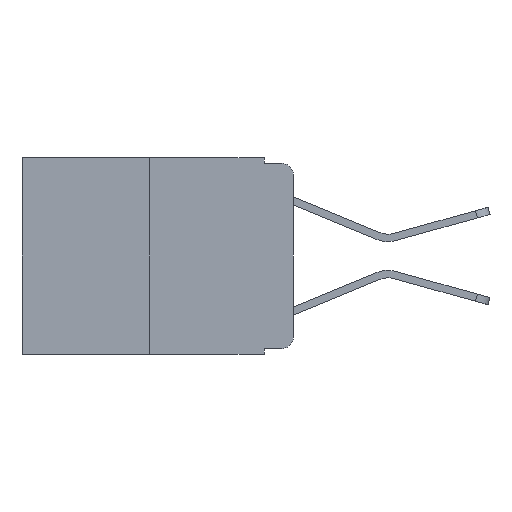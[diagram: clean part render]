
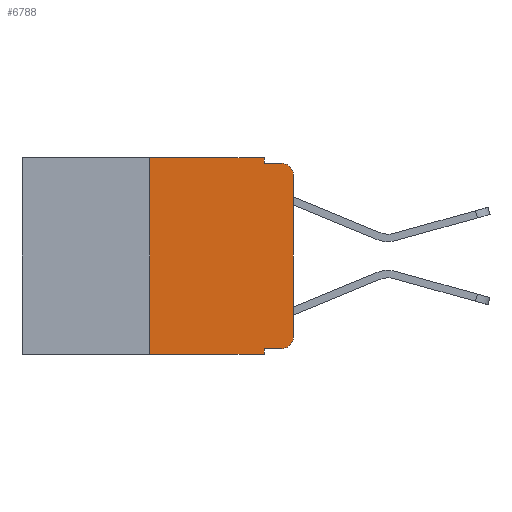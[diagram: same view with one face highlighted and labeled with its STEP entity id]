
A CAD part, left-side view. The second image highlights one B-rep face of the part: STEP entity #6788.
In plain terms, the highlighted planar face has unit normal (-1, 0, 0).
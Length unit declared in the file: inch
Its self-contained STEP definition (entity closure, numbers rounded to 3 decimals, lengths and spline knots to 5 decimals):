
#17 = DIRECTION ( 'NONE',  ( 1., 0., 0. ) ) ;
#64 = ORIENTED_EDGE ( 'NONE', *, *, #7757, .T. ) ;
#306 = CARTESIAN_POINT ( 'NONE',  ( 0., 0.02, -0.313 ) ) ;
#849 = ORIENTED_EDGE ( 'NONE', *, *, #4916, .T. ) ;
#918 = LINE ( 'NONE', #1607, #7375 ) ;
#1064 = AXIS2_PLACEMENT_3D ( 'NONE', #2397, #3170, #8493 ) ;
#1242 = DIRECTION ( 'NONE',  ( 0., -1., 0. ) ) ;
#1512 = EDGE_CURVE ( 'NONE', #9832, #6600, #7458, .T. ) ;
#1607 = CARTESIAN_POINT ( 'NONE',  ( 0., 0.473, 0. ) ) ;
#1700 = LINE ( 'NONE', #7410, #6364 ) ;
#1764 = DIRECTION ( 'NONE',  ( -1., 0., 0. ) ) ;
#1778 = ORIENTED_EDGE ( 'NONE', *, *, #9195, .F. ) ;
#2038 = LINE ( 'NONE', #7457, #3850 ) ;
#2186 = EDGE_CURVE ( 'NONE', #6170, #4249, #1700, .T. ) ;
#2193 = CARTESIAN_POINT ( 'NONE',  ( 0., 0.25, -0.343 ) ) ;
#2313 = VECTOR ( 'NONE', #8020, 39.37008 ) ;
#2341 = EDGE_CURVE ( 'NONE', #6851, #3588, #7324, .T. ) ;
#2349 = VERTEX_POINT ( 'NONE', #8734 ) ;
#2397 = CARTESIAN_POINT ( 'NONE',  ( 0., 0.02, -0.03 ) ) ;
#2400 = CARTESIAN_POINT ( 'NONE',  ( 0., 0.051, 0. ) ) ;
#2584 = CARTESIAN_POINT ( 'NONE',  ( 0., 0.051, 0. ) ) ;
#3016 = CARTESIAN_POINT ( 'NONE',  ( 0., 0.051, -0.01 ) ) ;
#3042 = DIRECTION ( 'NONE',  ( 0., -1., 0. ) ) ;
#3071 = ORIENTED_EDGE ( 'NONE', *, *, #1512, .T. ) ;
#3081 = DIRECTION ( 'NONE',  ( 0., -1., 0. ) ) ;
#3120 = CIRCLE ( 'NONE', #7916, 0.02 ) ;
#3170 = DIRECTION ( 'NONE',  ( -1., 0., 0. ) ) ;
#3588 = VERTEX_POINT ( 'NONE', #3016 ) ;
#3607 = CARTESIAN_POINT ( 'NONE',  ( 0., 0.051, -0.333 ) ) ;
#3850 = VECTOR ( 'NONE', #1242, 39.37008 ) ;
#3873 = AXIS2_PLACEMENT_3D ( 'NONE', #4579, #17, #6083 ) ;
#4003 = EDGE_CURVE ( 'NONE', #6170, #6740, #6093, .T. ) ;
#4177 = CARTESIAN_POINT ( 'NONE',  ( 0., 0.051, -0.333 ) ) ;
#4242 = ORIENTED_EDGE ( 'NONE', *, *, #4003, .T. ) ;
#4249 = VERTEX_POINT ( 'NONE', #7710 ) ;
#4347 = ORIENTED_EDGE ( 'NONE', *, *, #9548, .T. ) ;
#4456 = PLANE ( 'NONE',  #3873 ) ;
#4551 = VECTOR ( 'NONE', #4688, 39.37008 ) ;
#4579 = CARTESIAN_POINT ( 'NONE',  ( 0., 0.473, 0. ) ) ;
#4593 = ORIENTED_EDGE ( 'NONE', *, *, #8394, .F. ) ;
#4688 = DIRECTION ( 'NONE',  ( 0., 0., -1. ) ) ;
#4916 = EDGE_CURVE ( 'NONE', #9144, #8566, #8111, .T. ) ;
#4969 = DIRECTION ( 'NONE',  ( 0., -1., 0. ) ) ;
#5065 = CARTESIAN_POINT ( 'NONE',  ( 0., 0., 0. ) ) ;
#5389 = LINE ( 'NONE', #2584, #6111 ) ;
#5541 = EDGE_CURVE ( 'NONE', #4249, #6851, #918, .T. ) ;
#5925 = CARTESIAN_POINT ( 'NONE',  ( 0., 0.051, -0.343 ) ) ;
#6031 = FACE_OUTER_BOUND ( 'NONE', #6336, .T. ) ;
#6083 = DIRECTION ( 'NONE',  ( 0., 0., -1. ) ) ;
#6093 = LINE ( 'NONE', #7623, #6450 ) ;
#6111 = VECTOR ( 'NONE', #7241, 39.37008 ) ;
#6170 = VERTEX_POINT ( 'NONE', #2193 ) ;
#6336 = EDGE_LOOP ( 'NONE', ( #64, #849, #1778, #9250, #8814, #6541, #4242, #4593, #3071, #4347 ) ) ;
#6364 = VECTOR ( 'NONE', #6661, 39.37008 ) ;
#6450 = VECTOR ( 'NONE', #3042, 39.37008 ) ;
#6541 = ORIENTED_EDGE ( 'NONE', *, *, #2186, .F. ) ;
#6600 = VERTEX_POINT ( 'NONE', #8202 ) ;
#6661 = DIRECTION ( 'NONE',  ( 0., 0., 1. ) ) ;
#6740 = VERTEX_POINT ( 'NONE', #5925 ) ;
#6756 = CARTESIAN_POINT ( 'NONE',  ( 0., 0.051, 0. ) ) ;
#6788 = ADVANCED_FACE ( 'NONE', ( #6031 ), #4456, .F. ) ;
#6851 = VERTEX_POINT ( 'NONE', #6756 ) ;
#7241 = DIRECTION ( 'NONE',  ( 0., 0., -1. ) ) ;
#7324 = LINE ( 'NONE', #2400, #4551 ) ;
#7363 = CARTESIAN_POINT ( 'NONE',  ( 0., 0., -0.03 ) ) ;
#7375 = VECTOR ( 'NONE', #3081, 39.37008 ) ;
#7410 = CARTESIAN_POINT ( 'NONE',  ( 0., 0.25, 0. ) ) ;
#7457 = CARTESIAN_POINT ( 'NONE',  ( 0., 0.051, -0.01 ) ) ;
#7458 = LINE ( 'NONE', #4177, #8292 ) ;
#7578 = LINE ( 'NONE', #5065, #2313 ) ;
#7623 = CARTESIAN_POINT ( 'NONE',  ( 0., 0.473, -0.343 ) ) ;
#7710 = CARTESIAN_POINT ( 'NONE',  ( 0., 0.25, 0. ) ) ;
#7757 = EDGE_CURVE ( 'NONE', #2349, #9144, #7578, .T. ) ;
#7916 = AXIS2_PLACEMENT_3D ( 'NONE', #306, #1764, #9385 ) ;
#8020 = DIRECTION ( 'NONE',  ( 0., 0., 1. ) ) ;
#8111 = CIRCLE ( 'NONE', #1064, 0.02 ) ;
#8202 = CARTESIAN_POINT ( 'NONE',  ( 0., 0.02, -0.333 ) ) ;
#8292 = VECTOR ( 'NONE', #4969, 39.37008 ) ;
#8394 = EDGE_CURVE ( 'NONE', #9832, #6740, #5389, .T. ) ;
#8493 = DIRECTION ( 'NONE',  ( 0., 0., -1. ) ) ;
#8566 = VERTEX_POINT ( 'NONE', #9706 ) ;
#8734 = CARTESIAN_POINT ( 'NONE',  ( 0., 0., -0.313 ) ) ;
#8814 = ORIENTED_EDGE ( 'NONE', *, *, #5541, .F. ) ;
#9144 = VERTEX_POINT ( 'NONE', #7363 ) ;
#9195 = EDGE_CURVE ( 'NONE', #3588, #8566, #2038, .T. ) ;
#9250 = ORIENTED_EDGE ( 'NONE', *, *, #2341, .F. ) ;
#9385 = DIRECTION ( 'NONE',  ( 0., 0., -1. ) ) ;
#9548 = EDGE_CURVE ( 'NONE', #6600, #2349, #3120, .T. ) ;
#9706 = CARTESIAN_POINT ( 'NONE',  ( 0., 0.02, -0.01 ) ) ;
#9832 = VERTEX_POINT ( 'NONE', #3607 ) ;
